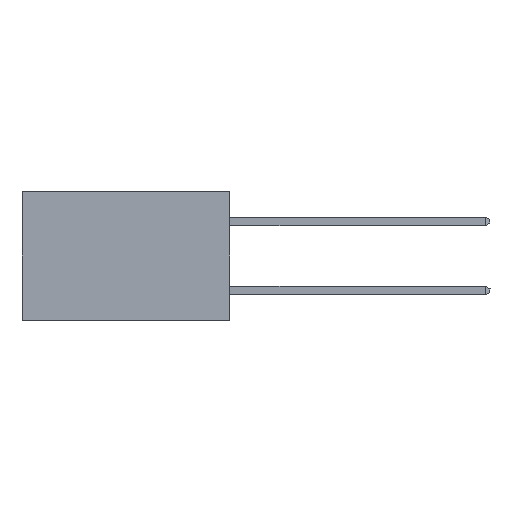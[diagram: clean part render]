
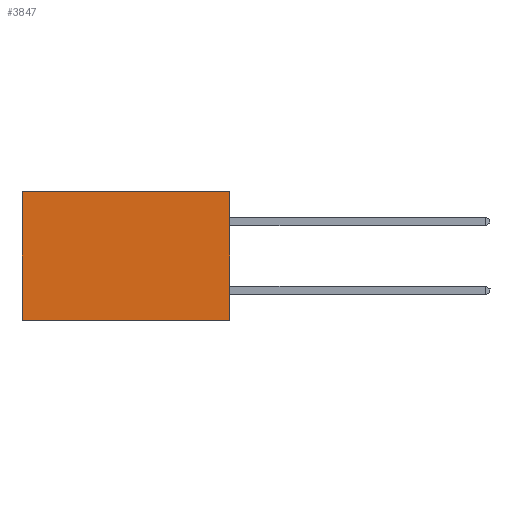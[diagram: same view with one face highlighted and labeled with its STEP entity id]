
A CAD part, left-side view. The second image highlights one B-rep face of the part: STEP entity #3847.
In plain terms, the highlighted planar face has unit normal (-1, 0, 0).
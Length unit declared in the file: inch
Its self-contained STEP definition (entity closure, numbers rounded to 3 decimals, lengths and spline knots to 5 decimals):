
#710 = AXIS2_PLACEMENT_3D ( 'NONE', #8389, #9345, #1813 ) ;
#880 = VERTEX_POINT ( 'NONE', #4859 ) ;
#1639 = VECTOR ( 'NONE', #13698, 39.37008 ) ;
#1684 = CARTESIAN_POINT ( 'NONE',  ( 0.298, 0.6, 0. ) ) ;
#1813 = DIRECTION ( 'NONE',  ( 0., 0., -1. ) ) ;
#2593 = EDGE_LOOP ( 'NONE', ( #8578, #13790, #8536, #4627 ) ) ;
#3038 = CARTESIAN_POINT ( 'NONE',  ( 0.298, 0., 0. ) ) ;
#3567 = EDGE_CURVE ( 'NONE', #5277, #880, #4736, .T. ) ;
#3847 = ADVANCED_FACE ( 'NONE', ( #14018 ), #3948, .F. ) ;
#3948 = PLANE ( 'NONE',  #710 ) ;
#4102 = EDGE_CURVE ( 'NONE', #11976, #5277, #11487, .T. ) ;
#4627 = ORIENTED_EDGE ( 'NONE', *, *, #4102, .T. ) ;
#4736 = LINE ( 'NONE', #1684, #1639 ) ;
#4859 = CARTESIAN_POINT ( 'NONE',  ( 0.298, 0.6, -0.37 ) ) ;
#5093 = VECTOR ( 'NONE', #10331, 39.37008 ) ;
#5277 = VERTEX_POINT ( 'NONE', #11165 ) ;
#5279 = EDGE_CURVE ( 'NONE', #11976, #13432, #9463, .T. ) ;
#6601 = LINE ( 'NONE', #7014, #5093 ) ;
#6881 = CARTESIAN_POINT ( 'NONE',  ( 0.298, 0., 0. ) ) ;
#6975 = DIRECTION ( 'NONE',  ( 0., 0., -1. ) ) ;
#7014 = CARTESIAN_POINT ( 'NONE',  ( 0.298, 0., -0.37 ) ) ;
#7370 = CARTESIAN_POINT ( 'NONE',  ( 0.298, 0., -0.37 ) ) ;
#7746 = VECTOR ( 'NONE', #6975, 39.37008 ) ;
#8389 = CARTESIAN_POINT ( 'NONE',  ( 0.298, 0., 0. ) ) ;
#8536 = ORIENTED_EDGE ( 'NONE', *, *, #5279, .F. ) ;
#8578 = ORIENTED_EDGE ( 'NONE', *, *, #3567, .T. ) ;
#8640 = VECTOR ( 'NONE', #9810, 39.37008 ) ;
#8771 = CARTESIAN_POINT ( 'NONE',  ( 0.298, 0., 0. ) ) ;
#9345 = DIRECTION ( 'NONE',  ( 1., 0., 0. ) ) ;
#9463 = LINE ( 'NONE', #6881, #7746 ) ;
#9810 = DIRECTION ( 'NONE',  ( 0., 1., 0. ) ) ;
#10331 = DIRECTION ( 'NONE',  ( 0., 1., 0. ) ) ;
#11165 = CARTESIAN_POINT ( 'NONE',  ( 0.298, 0.6, 0. ) ) ;
#11487 = LINE ( 'NONE', #8771, #8640 ) ;
#11976 = VERTEX_POINT ( 'NONE', #3038 ) ;
#12839 = EDGE_CURVE ( 'NONE', #13432, #880, #6601, .T. ) ;
#13432 = VERTEX_POINT ( 'NONE', #7370 ) ;
#13698 = DIRECTION ( 'NONE',  ( 0., 0., -1. ) ) ;
#13790 = ORIENTED_EDGE ( 'NONE', *, *, #12839, .F. ) ;
#14018 = FACE_OUTER_BOUND ( 'NONE', #2593, .T. ) ;
